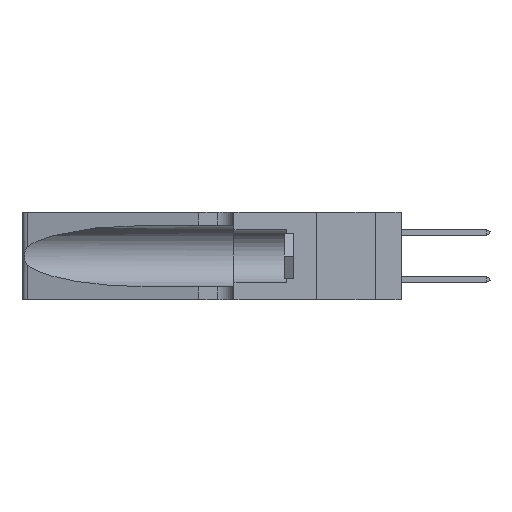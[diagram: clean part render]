
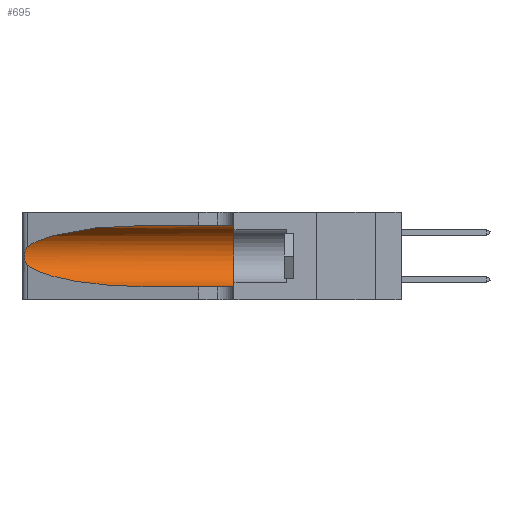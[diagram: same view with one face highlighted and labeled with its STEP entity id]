
A CAD part, left-side view. The second image highlights one B-rep face of the part: STEP entity #695.
In plain terms, the highlighted cylindrical face has radius 3.308 mm (diameter 6.617 mm), a partial arc.
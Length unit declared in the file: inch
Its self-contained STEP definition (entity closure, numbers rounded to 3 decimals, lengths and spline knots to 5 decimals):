
#349 =( BOUNDED_CURVE ( )  B_SPLINE_CURVE ( 3, ( #14511, #3075, #29007, #11753 ),
 .UNSPECIFIED., .F., .F. ) 
 B_SPLINE_CURVE_WITH_KNOTS ( ( 4, 4 ),
 ( 3.44316, 4.71239 ),
 .UNSPECIFIED. ) 
 CURVE ( )  GEOMETRIC_REPRESENTATION_ITEM ( )  RATIONAL_B_SPLINE_CURVE ( ( 1., 0.87, 0.87, 1. ) ) 
 REPRESENTATION_ITEM ( '' )  );
#695 = ADVANCED_FACE ( 'NONE', ( #31772 ), #16485, .F. ) ;
#1056 = DIRECTION ( 'NONE',  ( 0., -1., 0. ) ) ;
#1066 = CARTESIAN_POINT ( 'NONE',  ( 0.25555, 1.22994, 0.2215 ) ) ;
#1185 = CARTESIAN_POINT ( 'NONE',  ( 0.25639, 1.23184, 0.21858 ) ) ;
#1834 = ORIENTED_EDGE ( 'NONE', *, *, #32444, .T. ) ;
#2550 = CARTESIAN_POINT ( 'NONE',  ( 0.1305, 1.61858, 0.185 ) ) ;
#3075 = CARTESIAN_POINT ( 'NONE',  ( 0.2373, 1.15595, 0.08982 ) ) ;
#3385 = DIRECTION ( 'NONE',  ( 0., 1., 0. ) ) ;
#3667 = ORIENTED_EDGE ( 'NONE', *, *, #33889, .T. ) ;
#4144 = CARTESIAN_POINT ( 'NONE',  ( 0.25854, 1.2359, 0.20912 ) ) ;
#4328 = EDGE_CURVE ( 'NONE', #14513, #35969, #21360, .T. ) ;
#6065 = VECTOR ( 'NONE', #12797, 39.37008 ) ;
#7030 = CARTESIAN_POINT ( 'NONE',  ( 0.26075, 1.23896, 0.19203 ) ) ;
#7879 = CARTESIAN_POINT ( 'NONE',  ( 0.1305, 0.35, 0.05475 ) ) ;
#8694 = ORIENTED_EDGE ( 'NONE', *, *, #32270, .F. ) ;
#8885 = CIRCLE ( 'NONE', #20464, 0.13025 ) ;
#9341 = EDGE_LOOP ( 'NONE', ( #28392, #1834, #3667, #30746, #8694, #10494 ) ) ;
#9649 = CARTESIAN_POINT ( 'NONE',  ( 0.1305, 1.61858, 0.05475 ) ) ;
#9909 = CARTESIAN_POINT ( 'NONE',  ( 0.26017, 1.23833, 0.17102 ) ) ;
#9913 = CARTESIAN_POINT ( 'NONE',  ( 0.1305, 1.61858, 0.31525 ) ) ;
#10184 = CARTESIAN_POINT ( 'NONE',  ( 0.18966, 0.96281, 0.31525 ) ) ;
#10494 = ORIENTED_EDGE ( 'NONE', *, *, #4328, .F. ) ;
#11188 = VERTEX_POINT ( 'NONE', #35582 ) ;
#11753 = CARTESIAN_POINT ( 'NONE',  ( 0.1305, 0.72297, 0.05475 ) ) ;
#12759 = AXIS2_PLACEMENT_3D ( 'NONE', #2550, #22561, #22689 ) ;
#12794 = CARTESIAN_POINT ( 'NONE',  ( 0.25789, 1.23486, 0.15765 ) ) ;
#12797 = DIRECTION ( 'NONE',  ( 0., -1., 0. ) ) ;
#13581 = CARTESIAN_POINT ( 'NONE',  ( 0.2373, 1.15595, 0.28018 ) ) ;
#13749 = B_SPLINE_CURVE_WITH_KNOTS ( 'NONE', 3,
 ( #29802, #1066, #1185, #21365, #4144, #24254, #7030, #27149, #9909, #30050, #12794, #32895, #15706, #35786 ),
 .UNSPECIFIED., .F., .F.,
 ( 4, 2, 2, 2, 2, 2, 4 ),
 ( 0., 0.00027, 0.00053, 0.00107, 0.0016, 0.00187, 0.00214 ),
 .UNSPECIFIED. ) ;
#14511 = CARTESIAN_POINT ( 'NONE',  ( 0.25487, 1.22718, 0.14631 ) ) ;
#14513 = VERTEX_POINT ( 'NONE', #33493 ) ;
#15131 = CARTESIAN_POINT ( 'NONE',  ( 0.25487, 1.22718, 0.14631 ) ) ;
#15706 = CARTESIAN_POINT ( 'NONE',  ( 0.25555, 1.22993, 0.14849 ) ) ;
#16485 = CYLINDRICAL_SURFACE ( 'NONE', #12759, 0.13025 ) ;
#16627 = VERTEX_POINT ( 'NONE', #15131 ) ;
#17689 =( BOUNDED_CURVE ( )  B_SPLINE_CURVE ( 3, ( #27435, #10184, #13581, #33689 ),
 .UNSPECIFIED., .F., .T. ) 
 B_SPLINE_CURVE_WITH_KNOTS ( ( 4, 4 ),
 ( 1.5708, 2.84003 ),
 .UNSPECIFIED. ) 
 CURVE ( )  GEOMETRIC_REPRESENTATION_ITEM ( )  RATIONAL_B_SPLINE_CURVE ( ( 1., 0.87, 0.87, 1. ) ) 
 REPRESENTATION_ITEM ( '' )  );
#17850 = VERTEX_POINT ( 'NONE', #20346 ) ;
#20346 = CARTESIAN_POINT ( 'NONE',  ( 0.1305, 0.72297, 0.05475 ) ) ;
#20464 = AXIS2_PLACEMENT_3D ( 'NONE', #20627, #3385, #23500 ) ;
#20534 = EDGE_CURVE ( 'NONE', #17850, #21753, #23511, .T. ) ;
#20627 = CARTESIAN_POINT ( 'NONE',  ( 0.1305, 0.35, 0.185 ) ) ;
#21360 = LINE ( 'NONE', #9913, #6065 ) ;
#21365 = CARTESIAN_POINT ( 'NONE',  ( 0.25787, 1.23484, 0.2124 ) ) ;
#21753 = VERTEX_POINT ( 'NONE', #7879 ) ;
#22561 = DIRECTION ( 'NONE',  ( 0., -1., 0. ) ) ;
#22626 = VECTOR ( 'NONE', #1056, 39.37008 ) ;
#22689 = DIRECTION ( 'NONE',  ( 0., 0., -1. ) ) ;
#23500 = DIRECTION ( 'NONE',  ( 0., 0., 1. ) ) ;
#23511 = LINE ( 'NONE', #9649, #22626 ) ;
#24254 = CARTESIAN_POINT ( 'NONE',  ( 0.26018, 1.23835, 0.19895 ) ) ;
#27149 = CARTESIAN_POINT ( 'NONE',  ( 0.26075, 1.23896, 0.178 ) ) ;
#27435 = CARTESIAN_POINT ( 'NONE',  ( 0.1305, 0.72297, 0.31525 ) ) ;
#28392 = ORIENTED_EDGE ( 'NONE', *, *, #34814, .T. ) ;
#29007 = CARTESIAN_POINT ( 'NONE',  ( 0.18966, 0.96281, 0.05475 ) ) ;
#29802 = CARTESIAN_POINT ( 'NONE',  ( 0.25487, 1.22718, 0.22369 ) ) ;
#30050 = CARTESIAN_POINT ( 'NONE',  ( 0.25856, 1.23593, 0.16098 ) ) ;
#30129 = CARTESIAN_POINT ( 'NONE',  ( 0.1305, 0.35, 0.31525 ) ) ;
#30746 = ORIENTED_EDGE ( 'NONE', *, *, #20534, .T. ) ;
#31772 = FACE_OUTER_BOUND ( 'NONE', #9341, .T. ) ;
#32270 = EDGE_CURVE ( 'NONE', #35969, #21753, #8885, .T. ) ;
#32444 = EDGE_CURVE ( 'NONE', #11188, #16627, #13749, .T. ) ;
#32895 = CARTESIAN_POINT ( 'NONE',  ( 0.25639, 1.23186, 0.15144 ) ) ;
#33493 = CARTESIAN_POINT ( 'NONE',  ( 0.1305, 0.72297, 0.31525 ) ) ;
#33689 = CARTESIAN_POINT ( 'NONE',  ( 0.25487, 1.22718, 0.22369 ) ) ;
#33889 = EDGE_CURVE ( 'NONE', #16627, #17850, #349, .T. ) ;
#34814 = EDGE_CURVE ( 'NONE', #14513, #11188, #17689, .T. ) ;
#35582 = CARTESIAN_POINT ( 'NONE',  ( 0.25487, 1.22718, 0.22369 ) ) ;
#35786 = CARTESIAN_POINT ( 'NONE',  ( 0.25487, 1.22718, 0.14631 ) ) ;
#35969 = VERTEX_POINT ( 'NONE', #30129 ) ;
